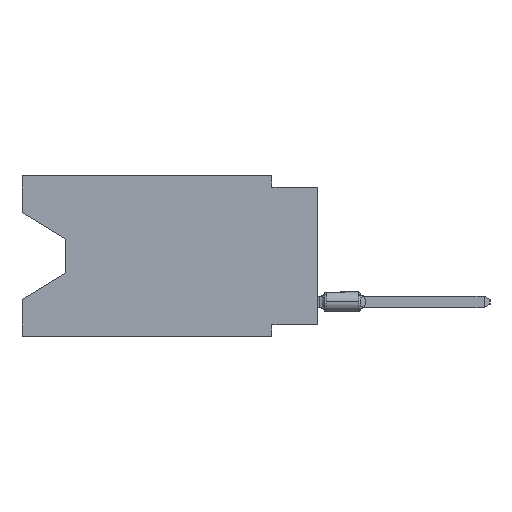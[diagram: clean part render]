
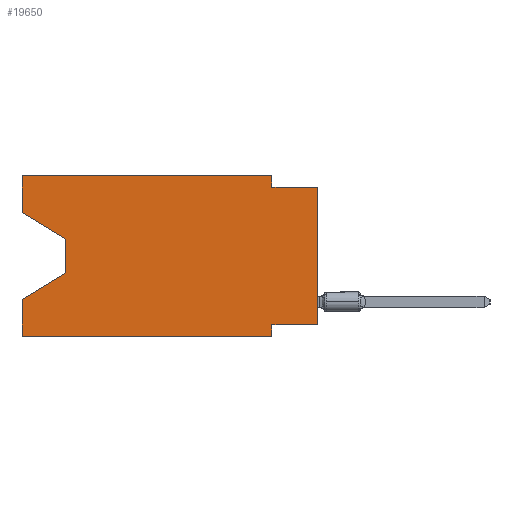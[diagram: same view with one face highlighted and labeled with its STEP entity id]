
A CAD part, left-side view. The second image highlights one B-rep face of the part: STEP entity #19650.
In plain terms, the highlighted planar face has unit normal (-1, 0, 0).
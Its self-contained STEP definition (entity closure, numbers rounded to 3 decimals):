
#156 = EDGE_CURVE ( 'NONE', #57861, #55762, #62294, .T. ) ;
#487 = VERTEX_POINT ( 'NONE', #49683 ) ;
#621 = PLANE ( 'NONE',  #25989 ) ;
#1055 = DIRECTION ( 'NONE',  ( 0., -0.855, -0.519 ) ) ;
#1926 = ORIENTED_EDGE ( 'NONE', *, *, #24034, .T. ) ;
#2203 = VECTOR ( 'NONE', #41065, 1000. ) ;
#2484 = CARTESIAN_POINT ( 'NONE',  ( 0., 0., -0.635 ) ) ;
#3643 = LINE ( 'NONE', #36496, #2203 ) ;
#3934 = VECTOR ( 'NONE', #35130, 1000. ) ;
#4063 = EDGE_CURVE ( 'NONE', #46571, #12998, #23801, .T. ) ;
#4243 = VERTEX_POINT ( 'NONE', #32390 ) ;
#4450 = EDGE_CURVE ( 'NONE', #57861, #57140, #59670, .T. ) ;
#4465 = VECTOR ( 'NONE', #64858, 1000. ) ;
#4558 = DIRECTION ( 'NONE',  ( 0., -1., 0. ) ) ;
#5003 = CARTESIAN_POINT ( 'NONE',  ( 0., 2.54, -8.89 ) ) ;
#6318 = LINE ( 'NONE', #27659, #50937 ) ;
#6564 = DIRECTION ( 'NONE',  ( 0., 0., -1. ) ) ;
#9247 = EDGE_CURVE ( 'NONE', #27825, #487, #25001, .T. ) ;
#11482 = DIRECTION ( 'NONE',  ( 1., 0., 0. ) ) ;
#11746 = DIRECTION ( 'NONE',  ( 0., 0., 1. ) ) ;
#12300 = CARTESIAN_POINT ( 'NONE',  ( 0., 0., -8.255 ) ) ;
#12439 = CARTESIAN_POINT ( 'NONE',  ( 0., 16.383, 0. ) ) ;
#12844 = VERTEX_POINT ( 'NONE', #21778 ) ;
#12998 = VERTEX_POINT ( 'NONE', #2484 ) ;
#14196 = ORIENTED_EDGE ( 'NONE', *, *, #4450, .F. ) ;
#14723 = CARTESIAN_POINT ( 'NONE',  ( 0., 16.383, -8.89 ) ) ;
#15105 = ORIENTED_EDGE ( 'NONE', *, *, #156, .T. ) ;
#16200 = VECTOR ( 'NONE', #67434, 1000. ) ;
#16773 = VECTOR ( 'NONE', #64384, 1000. ) ;
#18068 = ORIENTED_EDGE ( 'NONE', *, *, #9247, .F. ) ;
#18286 = ORIENTED_EDGE ( 'NONE', *, *, #46163, .F. ) ;
#19448 = VECTOR ( 'NONE', #39869, 1000. ) ;
#19650 = ADVANCED_FACE ( 'NONE', ( #48207 ), #621, .F. ) ;
#20347 = CARTESIAN_POINT ( 'NONE',  ( 0., 2.54, 0. ) ) ;
#21451 = LINE ( 'NONE', #5003, #24974 ) ;
#21778 = CARTESIAN_POINT ( 'NONE',  ( 0., 13.97, -3.505 ) ) ;
#22506 = VECTOR ( 'NONE', #45522, 1000. ) ;
#23801 = LINE ( 'NONE', #25071, #58065 ) ;
#24034 = EDGE_CURVE ( 'NONE', #32206, #12998, #66078, .T. ) ;
#24206 = LINE ( 'NONE', #46202, #22506 ) ;
#24974 = VECTOR ( 'NONE', #42070, 1000. ) ;
#25001 = LINE ( 'NONE', #66958, #3934 ) ;
#25071 = CARTESIAN_POINT ( 'NONE',  ( 0., 0., -0.635 ) ) ;
#25989 = AXIS2_PLACEMENT_3D ( 'NONE', #43289, #11482, #6564 ) ;
#27127 = CARTESIAN_POINT ( 'NONE',  ( 0., 2.54, 0. ) ) ;
#27659 = CARTESIAN_POINT ( 'NONE',  ( 0., 16.383, -2.038 ) ) ;
#27711 = EDGE_CURVE ( 'NONE', #61388, #46571, #49833, .T. ) ;
#27825 = VERTEX_POINT ( 'NONE', #50520 ) ;
#29016 = ORIENTED_EDGE ( 'NONE', *, *, #43683, .F. ) ;
#29049 = DIRECTION ( 'NONE',  ( 0., -1., 0. ) ) ;
#30470 = CARTESIAN_POINT ( 'NONE',  ( 0., 2.54, -0.635 ) ) ;
#32131 = CARTESIAN_POINT ( 'NONE',  ( 0., 13.97, -5.385 ) ) ;
#32206 = VERTEX_POINT ( 'NONE', #42359 ) ;
#32390 = CARTESIAN_POINT ( 'NONE',  ( 0., 2.54, -8.255 ) ) ;
#33589 = EDGE_CURVE ( 'NONE', #32206, #4243, #44107, .T. ) ;
#34004 = EDGE_LOOP ( 'NONE', ( #56840, #50585, #60923, #14196, #15105, #18286, #50189, #1926, #36354, #48547, #29016, #18068 ) ) ;
#35130 = DIRECTION ( 'NONE',  ( 0., 0., 1. ) ) ;
#36354 = ORIENTED_EDGE ( 'NONE', *, *, #4063, .F. ) ;
#36496 = CARTESIAN_POINT ( 'NONE',  ( 0., 13.97, -3.505 ) ) ;
#39869 = DIRECTION ( 'NONE',  ( 0., 1., 0. ) ) ;
#41065 = DIRECTION ( 'NONE',  ( 0., 0., -1. ) ) ;
#42070 = DIRECTION ( 'NONE',  ( 0., 0., -1. ) ) ;
#42359 = CARTESIAN_POINT ( 'NONE',  ( 0., 0., -8.255 ) ) ;
#43036 = CARTESIAN_POINT ( 'NONE',  ( 0., 16.383, 0. ) ) ;
#43289 = CARTESIAN_POINT ( 'NONE',  ( 0., 16.383, 0. ) ) ;
#43683 = EDGE_CURVE ( 'NONE', #487, #61388, #60198, .T. ) ;
#44082 = VERTEX_POINT ( 'NONE', #32131 ) ;
#44107 = LINE ( 'NONE', #12300, #19448 ) ;
#45522 = DIRECTION ( 'NONE',  ( 0., 0.855, -0.519 ) ) ;
#46163 = EDGE_CURVE ( 'NONE', #4243, #55762, #21451, .T. ) ;
#46202 = CARTESIAN_POINT ( 'NONE',  ( 0., 13.97, -5.385 ) ) ;
#46571 = VERTEX_POINT ( 'NONE', #30470 ) ;
#46796 = CARTESIAN_POINT ( 'NONE',  ( 0., 16.383, -6.852 ) ) ;
#48207 = FACE_OUTER_BOUND ( 'NONE', #34004, .T. ) ;
#48547 = ORIENTED_EDGE ( 'NONE', *, *, #27711, .F. ) ;
#48632 = EDGE_CURVE ( 'NONE', #27825, #12844, #6318, .T. ) ;
#49683 = CARTESIAN_POINT ( 'NONE',  ( 0., 16.383, 0. ) ) ;
#49833 = LINE ( 'NONE', #27127, #4465 ) ;
#50189 = ORIENTED_EDGE ( 'NONE', *, *, #33589, .F. ) ;
#50520 = CARTESIAN_POINT ( 'NONE',  ( 0., 16.383, -2.038 ) ) ;
#50585 = ORIENTED_EDGE ( 'NONE', *, *, #64623, .T. ) ;
#50937 = VECTOR ( 'NONE', #1055, 1000. ) ;
#51727 = CARTESIAN_POINT ( 'NONE',  ( 0., 0., 0. ) ) ;
#55443 = VECTOR ( 'NONE', #4558, 1000. ) ;
#55762 = VERTEX_POINT ( 'NONE', #60337 ) ;
#55886 = VECTOR ( 'NONE', #11746, 1000. ) ;
#56840 = ORIENTED_EDGE ( 'NONE', *, *, #48632, .T. ) ;
#57140 = VERTEX_POINT ( 'NONE', #46796 ) ;
#57861 = VERTEX_POINT ( 'NONE', #60961 ) ;
#58065 = VECTOR ( 'NONE', #29049, 1000. ) ;
#59670 = LINE ( 'NONE', #12439, #55886 ) ;
#60198 = LINE ( 'NONE', #43036, #16773 ) ;
#60337 = CARTESIAN_POINT ( 'NONE',  ( 0., 2.54, -8.89 ) ) ;
#60923 = ORIENTED_EDGE ( 'NONE', *, *, #67304, .T. ) ;
#60961 = CARTESIAN_POINT ( 'NONE',  ( 0., 16.383, -8.89 ) ) ;
#61388 = VERTEX_POINT ( 'NONE', #20347 ) ;
#62294 = LINE ( 'NONE', #14723, #55443 ) ;
#64384 = DIRECTION ( 'NONE',  ( 0., -1., 0. ) ) ;
#64623 = EDGE_CURVE ( 'NONE', #12844, #44082, #3643, .T. ) ;
#64858 = DIRECTION ( 'NONE',  ( 0., 0., -1. ) ) ;
#66078 = LINE ( 'NONE', #51727, #16200 ) ;
#66958 = CARTESIAN_POINT ( 'NONE',  ( 0., 16.383, 0. ) ) ;
#67304 = EDGE_CURVE ( 'NONE', #44082, #57140, #24206, .T. ) ;
#67434 = DIRECTION ( 'NONE',  ( 0., 0., 1. ) ) ;
